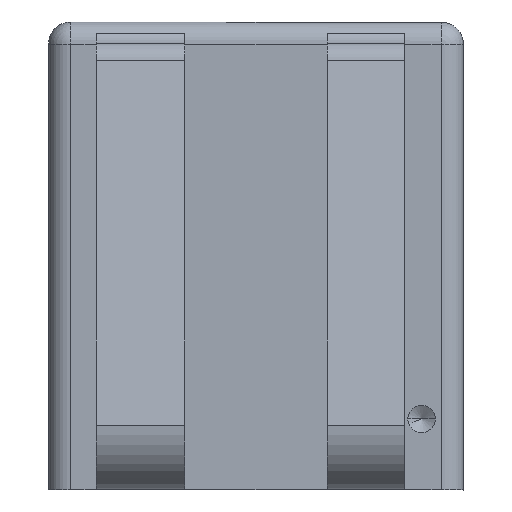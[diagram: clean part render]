
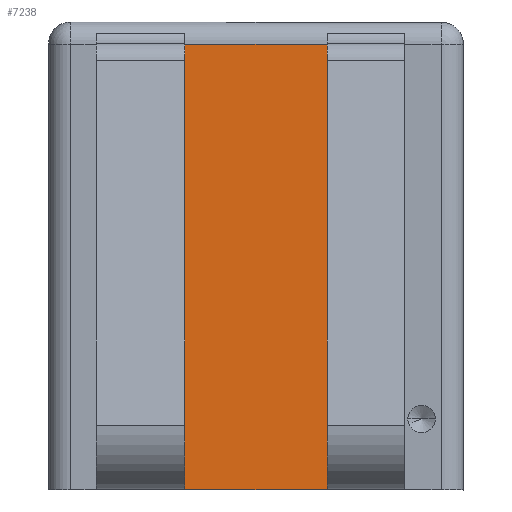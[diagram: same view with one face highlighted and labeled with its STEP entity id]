
A CAD part, front view. The second image highlights one B-rep face of the part: STEP entity #7238.
In plain terms, the highlighted planar face has unit normal (0, -1, 0).
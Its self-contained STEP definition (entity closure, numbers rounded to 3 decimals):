
#134 = CARTESIAN_POINT ( 'NONE',  ( -24.701, -47.706, 236.358 ) ) ;
#500 = FACE_OUTER_BOUND ( 'NONE', #9134, .T. ) ;
#567 = CARTESIAN_POINT ( 'NONE',  ( 25.299, -47.706, 198.094 ) ) ;
#643 = VERTEX_POINT ( 'NONE', #7896 ) ;
#1188 = DIRECTION ( 'NONE',  ( 0., 0., 1. ) ) ;
#1310 = VECTOR ( 'NONE', #1188, 1000. ) ;
#1361 = DIRECTION ( 'NONE',  ( 0., 0., 1. ) ) ;
#1417 = ORIENTED_EDGE ( 'NONE', *, *, #5724, .F. ) ;
#1555 = CARTESIAN_POINT ( 'NONE',  ( 18.39, -47.706, 196.506 ) ) ;
#1792 = CARTESIAN_POINT ( 'NONE',  ( 5.69, -47.706, 236.358 ) ) ;
#1859 = VECTOR ( 'NONE', #6149, 1000. ) ;
#2097 = VECTOR ( 'NONE', #2499, 1000. ) ;
#2358 = CARTESIAN_POINT ( 'NONE',  ( 18.39, -47.706, 196.506 ) ) ;
#2499 = DIRECTION ( 'NONE',  ( 1., 0., 0. ) ) ;
#2551 = EDGE_CURVE ( 'NONE', #8631, #643, #5817, .T. ) ;
#3320 = ORIENTED_EDGE ( 'NONE', *, *, #9093, .F. ) ;
#3429 = LINE ( 'NONE', #5933, #1310 ) ;
#3632 = EDGE_CURVE ( 'NONE', #643, #6926, #3429, .T. ) ;
#4716 = DIRECTION ( 'NONE',  ( 0., 0., -1. ) ) ;
#5314 = PLANE ( 'NONE',  #7512 ) ;
#5529 = CARTESIAN_POINT ( 'NONE',  ( 5.69, -47.706, 196.506 ) ) ;
#5624 = LINE ( 'NONE', #2358, #7967 ) ;
#5724 = EDGE_CURVE ( 'NONE', #10209, #8631, #5624, .T. ) ;
#5817 = LINE ( 'NONE', #5529, #1859 ) ;
#5933 = CARTESIAN_POINT ( 'NONE',  ( 5.69, -47.706, 230.542 ) ) ;
#6104 = DIRECTION ( 'NONE',  ( 0., 1., 0. ) ) ;
#6149 = DIRECTION ( 'NONE',  ( -1., 0., 0. ) ) ;
#6301 = CARTESIAN_POINT ( 'NONE',  ( 18.39, -47.706, 236.358 ) ) ;
#6926 = VERTEX_POINT ( 'NONE', #1792 ) ;
#7238 = ADVANCED_FACE ( 'NONE', ( #500 ), #5314, .F. ) ;
#7512 = AXIS2_PLACEMENT_3D ( 'NONE', #567, #6104, #1361 ) ;
#7896 = CARTESIAN_POINT ( 'NONE',  ( 5.69, -47.706, 196.506 ) ) ;
#7967 = VECTOR ( 'NONE', #4716, 1000. ) ;
#8012 = ORIENTED_EDGE ( 'NONE', *, *, #3632, .F. ) ;
#8631 = VERTEX_POINT ( 'NONE', #1555 ) ;
#9093 = EDGE_CURVE ( 'NONE', #6926, #10209, #10005, .T. ) ;
#9134 = EDGE_LOOP ( 'NONE', ( #1417, #3320, #8012, #9927 ) ) ;
#9927 = ORIENTED_EDGE ( 'NONE', *, *, #2551, .F. ) ;
#10005 = LINE ( 'NONE', #134, #2097 ) ;
#10209 = VERTEX_POINT ( 'NONE', #6301 ) ;
